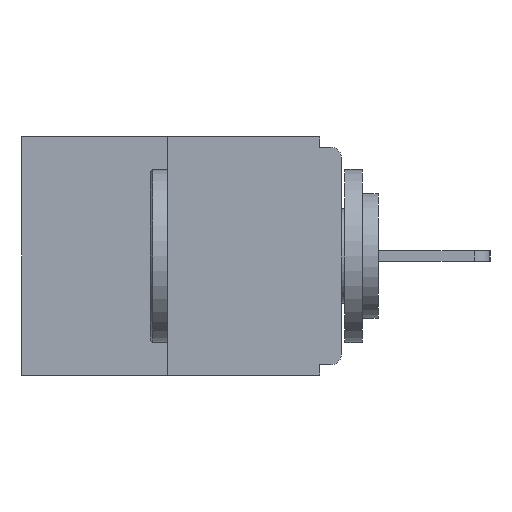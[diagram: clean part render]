
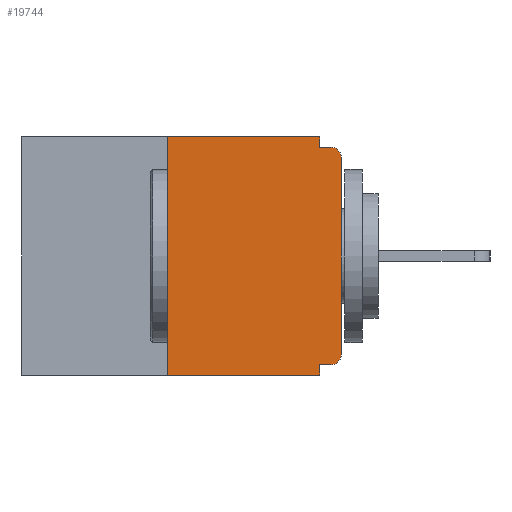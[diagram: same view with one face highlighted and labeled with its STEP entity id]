
A CAD part, left-side view. The second image highlights one B-rep face of the part: STEP entity #19744.
In plain terms, the highlighted planar face has unit normal (-1, 0, 0).
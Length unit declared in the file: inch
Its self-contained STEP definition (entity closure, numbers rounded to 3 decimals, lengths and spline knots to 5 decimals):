
#323 = LINE ( 'NONE', #17947, #4278 ) ;
#527 = CARTESIAN_POINT ( 'NONE',  ( 0., 0.015, -0.313 ) ) ;
#549 = FACE_OUTER_BOUND ( 'NONE', #1599, .T. ) ;
#889 = EDGE_CURVE ( 'NONE', #8279, #2133, #7391, .T. ) ;
#1126 = LINE ( 'NONE', #3498, #9530 ) ;
#1220 = CARTESIAN_POINT ( 'NONE',  ( 0., 0., -0.328 ) ) ;
#1599 = EDGE_LOOP ( 'NONE', ( #18196, #10377, #19178, #2544, #7578, #11894, #16061, #8093, #12419, #8321 ) ) ;
#1873 = DIRECTION ( 'NONE',  ( 0., 1., 0. ) ) ;
#2061 = DIRECTION ( 'NONE',  ( 0., 0., -1. ) ) ;
#2085 = CARTESIAN_POINT ( 'NONE',  ( 0., 0.015, -0.015 ) ) ;
#2133 = VERTEX_POINT ( 'NONE', #20193 ) ;
#2230 = DIRECTION ( 'NONE',  ( 0., 0., -1. ) ) ;
#2329 = CARTESIAN_POINT ( 'NONE',  ( 0., 0.25, 0. ) ) ;
#2509 = VERTEX_POINT ( 'NONE', #11156 ) ;
#2544 = ORIENTED_EDGE ( 'NONE', *, *, #11902, .F. ) ;
#2797 = LINE ( 'NONE', #12857, #11144 ) ;
#2888 = CARTESIAN_POINT ( 'NONE',  ( 0., 0.25, -0.343 ) ) ;
#2978 = CARTESIAN_POINT ( 'NONE',  ( 0., 0.031, -0.328 ) ) ;
#3217 = LINE ( 'NONE', #3791, #11560 ) ;
#3498 = CARTESIAN_POINT ( 'NONE',  ( 0., 0., -0.015 ) ) ;
#3573 = DIRECTION ( 'NONE',  ( 0., -1., 0. ) ) ;
#3683 = DIRECTION ( 'NONE',  ( 0., 0., 1. ) ) ;
#3791 = CARTESIAN_POINT ( 'NONE',  ( 0., 0., 0. ) ) ;
#4278 = VECTOR ( 'NONE', #8468, 39.37008 ) ;
#4307 = VERTEX_POINT ( 'NONE', #2085 ) ;
#4582 = DIRECTION ( 'NONE',  ( 0., 0., 1. ) ) ;
#4622 = EDGE_CURVE ( 'NONE', #14246, #14129, #20780, .T. ) ;
#5415 = CARTESIAN_POINT ( 'NONE',  ( 0., 0.031, -0.343 ) ) ;
#6041 = AXIS2_PLACEMENT_3D ( 'NONE', #7092, #12021, #2061 ) ;
#6416 = EDGE_CURVE ( 'NONE', #11274, #2509, #3217, .T. ) ;
#6502 = AXIS2_PLACEMENT_3D ( 'NONE', #8250, #19256, #9884 ) ;
#7092 = CARTESIAN_POINT ( 'NONE',  ( 0., 0.46, 0. ) ) ;
#7352 = DIRECTION ( 'NONE',  ( 0., 0., -1. ) ) ;
#7391 = LINE ( 'NONE', #8615, #10190 ) ;
#7518 = DIRECTION ( 'NONE',  ( 0., -1., 0. ) ) ;
#7578 = ORIENTED_EDGE ( 'NONE', *, *, #4622, .F. ) ;
#8093 = ORIENTED_EDGE ( 'NONE', *, *, #12878, .T. ) ;
#8250 = CARTESIAN_POINT ( 'NONE',  ( 0., 0.015, -0.03 ) ) ;
#8279 = VERTEX_POINT ( 'NONE', #18587 ) ;
#8321 = ORIENTED_EDGE ( 'NONE', *, *, #889, .F. ) ;
#8468 = DIRECTION ( 'NONE',  ( 0., -1., 0. ) ) ;
#8615 = CARTESIAN_POINT ( 'NONE',  ( 0., 0.031, 0. ) ) ;
#8619 = DIRECTION ( 'NONE',  ( 0., 0., -1. ) ) ;
#9302 = VECTOR ( 'NONE', #1873, 39.37008 ) ;
#9530 = VECTOR ( 'NONE', #3573, 39.37008 ) ;
#9884 = DIRECTION ( 'NONE',  ( 0., 0., -1. ) ) ;
#10190 = VECTOR ( 'NONE', #8619, 39.37008 ) ;
#10377 = ORIENTED_EDGE ( 'NONE', *, *, #15809, .F. ) ;
#11144 = VECTOR ( 'NONE', #4582, 39.37008 ) ;
#11156 = CARTESIAN_POINT ( 'NONE',  ( 0., 0., -0.03 ) ) ;
#11274 = VERTEX_POINT ( 'NONE', #16825 ) ;
#11560 = VECTOR ( 'NONE', #3683, 39.37008 ) ;
#11866 = EDGE_CURVE ( 'NONE', #14246, #11274, #19393, .T. ) ;
#11894 = ORIENTED_EDGE ( 'NONE', *, *, #11866, .T. ) ;
#11902 = EDGE_CURVE ( 'NONE', #14129, #12971, #18412, .T. ) ;
#12021 = DIRECTION ( 'NONE',  ( 1., 0., 0. ) ) ;
#12205 = DIRECTION ( 'NONE',  ( -1., 0., 0. ) ) ;
#12419 = ORIENTED_EDGE ( 'NONE', *, *, #17548, .F. ) ;
#12857 = CARTESIAN_POINT ( 'NONE',  ( 0., 0.25, 0. ) ) ;
#12878 = EDGE_CURVE ( 'NONE', #2509, #4307, #18802, .T. ) ;
#12971 = VERTEX_POINT ( 'NONE', #5415 ) ;
#13938 = VECTOR ( 'NONE', #7518, 39.37008 ) ;
#13941 = EDGE_CURVE ( 'NONE', #16486, #8279, #18001, .T. ) ;
#14129 = VERTEX_POINT ( 'NONE', #2978 ) ;
#14246 = VERTEX_POINT ( 'NONE', #16290 ) ;
#14571 = VERTEX_POINT ( 'NONE', #2888 ) ;
#15491 = CARTESIAN_POINT ( 'NONE',  ( 0., 0.46, 0. ) ) ;
#15809 = EDGE_CURVE ( 'NONE', #14571, #16486, #2797, .T. ) ;
#16061 = ORIENTED_EDGE ( 'NONE', *, *, #6416, .T. ) ;
#16201 = VECTOR ( 'NONE', #7352, 39.37008 ) ;
#16290 = CARTESIAN_POINT ( 'NONE',  ( 0., 0.015, -0.328 ) ) ;
#16486 = VERTEX_POINT ( 'NONE', #2329 ) ;
#16638 = PLANE ( 'NONE',  #6041 ) ;
#16690 = AXIS2_PLACEMENT_3D ( 'NONE', #527, #12205, #2230 ) ;
#16825 = CARTESIAN_POINT ( 'NONE',  ( 0., 0., -0.313 ) ) ;
#17548 = EDGE_CURVE ( 'NONE', #2133, #4307, #1126, .T. ) ;
#17947 = CARTESIAN_POINT ( 'NONE',  ( 0., 0.46, -0.343 ) ) ;
#17980 = EDGE_CURVE ( 'NONE', #14571, #12971, #323, .T. ) ;
#18001 = LINE ( 'NONE', #15491, #13938 ) ;
#18196 = ORIENTED_EDGE ( 'NONE', *, *, #13941, .F. ) ;
#18412 = LINE ( 'NONE', #19975, #16201 ) ;
#18587 = CARTESIAN_POINT ( 'NONE',  ( 0., 0.031, 0. ) ) ;
#18802 = CIRCLE ( 'NONE', #6502, 0.015 ) ;
#19178 = ORIENTED_EDGE ( 'NONE', *, *, #17980, .T. ) ;
#19256 = DIRECTION ( 'NONE',  ( -1., 0., 0. ) ) ;
#19393 = CIRCLE ( 'NONE', #16690, 0.015 ) ;
#19744 = ADVANCED_FACE ( 'NONE', ( #549 ), #16638, .F. ) ;
#19975 = CARTESIAN_POINT ( 'NONE',  ( 0., 0.031, -0.343 ) ) ;
#20193 = CARTESIAN_POINT ( 'NONE',  ( 0., 0.031, -0.015 ) ) ;
#20780 = LINE ( 'NONE', #1220, #9302 ) ;
